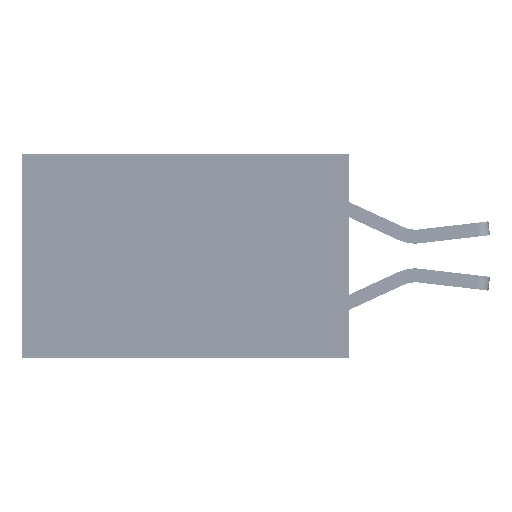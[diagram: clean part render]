
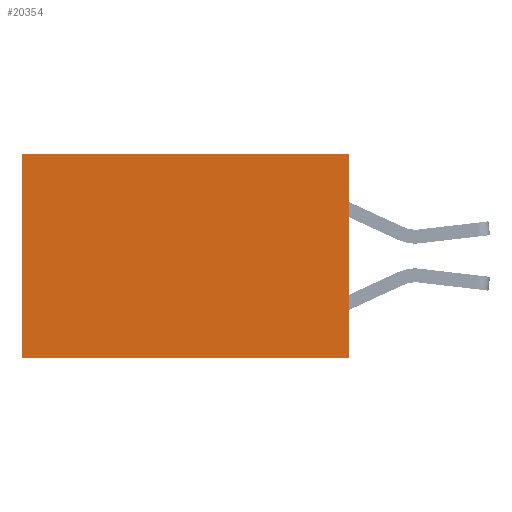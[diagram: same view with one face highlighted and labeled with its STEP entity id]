
A CAD part, left-side view. The second image highlights one B-rep face of the part: STEP entity #20354.
In plain terms, the highlighted planar face has unit normal (-1, 0, 0).
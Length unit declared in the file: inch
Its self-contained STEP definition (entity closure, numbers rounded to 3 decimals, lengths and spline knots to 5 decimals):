
#102 = VERTEX_POINT ( 'NONE', #3269 ) ;
#1640 = EDGE_LOOP ( 'NONE', ( #28164, #31705, #11642, #4911 ) ) ;
#3212 = DIRECTION ( 'NONE',  ( 0., 0., -1. ) ) ;
#3269 = CARTESIAN_POINT ( 'NONE',  ( 0.277, 0., -0.37 ) ) ;
#4005 = EDGE_CURVE ( 'NONE', #6423, #12271, #6961, .T. ) ;
#4898 = EDGE_CURVE ( 'NONE', #6423, #102, #11633, .T. ) ;
#4911 = ORIENTED_EDGE ( 'NONE', *, *, #4005, .T. ) ;
#5011 = EDGE_CURVE ( 'NONE', #12271, #28977, #9292, .T. ) ;
#6423 = VERTEX_POINT ( 'NONE', #12861 ) ;
#6961 = LINE ( 'NONE', #27483, #30965 ) ;
#8628 = LINE ( 'NONE', #15335, #27617 ) ;
#9104 = FACE_OUTER_BOUND ( 'NONE', #1640, .T. ) ;
#9292 = LINE ( 'NONE', #13537, #30571 ) ;
#11633 = LINE ( 'NONE', #17545, #32093 ) ;
#11642 = ORIENTED_EDGE ( 'NONE', *, *, #4898, .F. ) ;
#12271 = VERTEX_POINT ( 'NONE', #19306 ) ;
#12861 = CARTESIAN_POINT ( 'NONE',  ( 0.277, 0., 0. ) ) ;
#13537 = CARTESIAN_POINT ( 'NONE',  ( 0.277, 0.59, -0.37 ) ) ;
#13748 = DIRECTION ( 'NONE',  ( 0., 0., -1. ) ) ;
#15335 = CARTESIAN_POINT ( 'NONE',  ( 0.277, 0., -0.37 ) ) ;
#17545 = CARTESIAN_POINT ( 'NONE',  ( 0.277, 0., -0.37 ) ) ;
#17628 = DIRECTION ( 'NONE',  ( 0., 0., -1. ) ) ;
#18121 = DIRECTION ( 'NONE',  ( 1., 0., 0. ) ) ;
#18825 = CARTESIAN_POINT ( 'NONE',  ( 0.277, 0.59, -0.37 ) ) ;
#19306 = CARTESIAN_POINT ( 'NONE',  ( 0.277, 0.59, 0. ) ) ;
#20354 = ADVANCED_FACE ( 'NONE', ( #9104 ), #27972, .F. ) ;
#22827 = DIRECTION ( 'NONE',  ( 0., 1., 0. ) ) ;
#23017 = CARTESIAN_POINT ( 'NONE',  ( 0.277, 0., -0.37 ) ) ;
#25252 = AXIS2_PLACEMENT_3D ( 'NONE', #23017, #18121, #3212 ) ;
#27483 = CARTESIAN_POINT ( 'NONE',  ( 0.277, 0., 0. ) ) ;
#27617 = VECTOR ( 'NONE', #22827, 39.37008 ) ;
#27972 = PLANE ( 'NONE',  #25252 ) ;
#28164 = ORIENTED_EDGE ( 'NONE', *, *, #5011, .T. ) ;
#28379 = DIRECTION ( 'NONE',  ( 0., 1., 0. ) ) ;
#28977 = VERTEX_POINT ( 'NONE', #18825 ) ;
#30571 = VECTOR ( 'NONE', #13748, 39.37008 ) ;
#30965 = VECTOR ( 'NONE', #28379, 39.37008 ) ;
#31202 = EDGE_CURVE ( 'NONE', #102, #28977, #8628, .T. ) ;
#31705 = ORIENTED_EDGE ( 'NONE', *, *, #31202, .F. ) ;
#32093 = VECTOR ( 'NONE', #17628, 39.37008 ) ;
